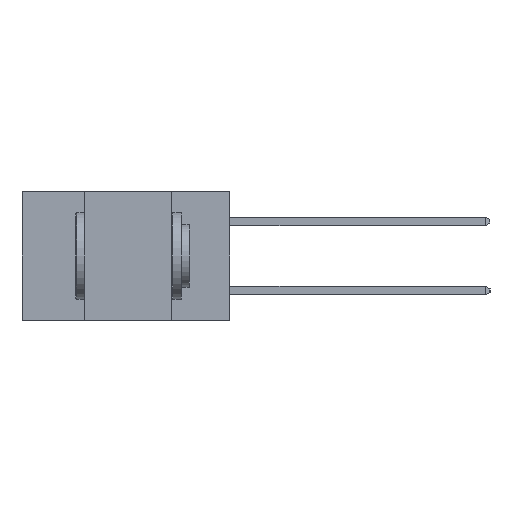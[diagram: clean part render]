
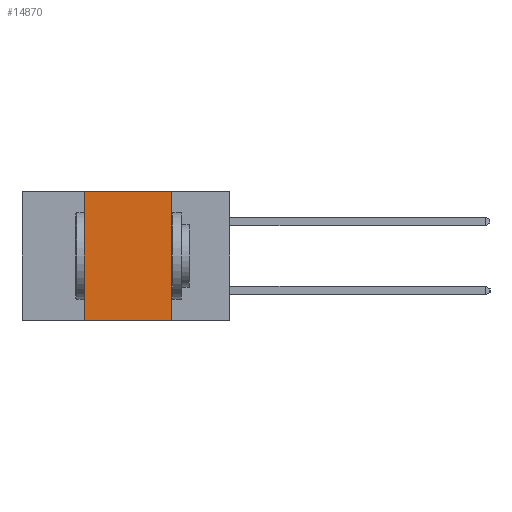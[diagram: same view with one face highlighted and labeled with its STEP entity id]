
A CAD part, left-side view. The second image highlights one B-rep face of the part: STEP entity #14870.
In plain terms, the highlighted planar face has unit normal (-1, 0, 0).
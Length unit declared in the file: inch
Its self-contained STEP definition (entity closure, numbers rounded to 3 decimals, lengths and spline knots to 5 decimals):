
#136 = CARTESIAN_POINT ( 'NONE',  ( 0., 0.6, 0. ) ) ;
#199 = LINE ( 'NONE', #8863, #11167 ) ;
#1555 = DIRECTION ( 'NONE',  ( 0., -1., 0. ) ) ;
#1939 = DIRECTION ( 'NONE',  ( 0., -1., 0. ) ) ;
#2019 = DIRECTION ( 'NONE',  ( 1., 0., 0. ) ) ;
#3711 = CARTESIAN_POINT ( 'NONE',  ( 0., 0.17, -0.37 ) ) ;
#3744 = ORIENTED_EDGE ( 'NONE', *, *, #12879, .F. ) ;
#4178 = FACE_OUTER_BOUND ( 'NONE', #18629, .T. ) ;
#4414 = LINE ( 'NONE', #15248, #24496 ) ;
#4954 = EDGE_CURVE ( 'NONE', #12142, #15135, #199, .T. ) ;
#5707 = CARTESIAN_POINT ( 'NONE',  ( 0., 0.17, 0. ) ) ;
#8863 = CARTESIAN_POINT ( 'NONE',  ( 0., 0.42, -0.37 ) ) ;
#8982 = LINE ( 'NONE', #3711, #13628 ) ;
#10090 = CARTESIAN_POINT ( 'NONE',  ( 0., 0.17, -0.37 ) ) ;
#10210 = EDGE_CURVE ( 'NONE', #12142, #16918, #4414, .T. ) ;
#10242 = AXIS2_PLACEMENT_3D ( 'NONE', #136, #2019, #15720 ) ;
#11167 = VECTOR ( 'NONE', #25030, 39.37008 ) ;
#11787 = PLANE ( 'NONE',  #10242 ) ;
#12142 = VERTEX_POINT ( 'NONE', #20817 ) ;
#12879 = EDGE_CURVE ( 'NONE', #15135, #16781, #23466, .T. ) ;
#13587 = ORIENTED_EDGE ( 'NONE', *, *, #18088, .F. ) ;
#13628 = VECTOR ( 'NONE', #15483, 39.37008 ) ;
#14186 = ORIENTED_EDGE ( 'NONE', *, *, #4954, .F. ) ;
#14870 = ADVANCED_FACE ( 'NONE', ( #4178 ), #11787, .F. ) ;
#15135 = VERTEX_POINT ( 'NONE', #24052 ) ;
#15248 = CARTESIAN_POINT ( 'NONE',  ( 0., 0.6, -0.37 ) ) ;
#15483 = DIRECTION ( 'NONE',  ( 0., 0., -1. ) ) ;
#15720 = DIRECTION ( 'NONE',  ( 0., 0., -1. ) ) ;
#16781 = VERTEX_POINT ( 'NONE', #5707 ) ;
#16918 = VERTEX_POINT ( 'NONE', #10090 ) ;
#17583 = CARTESIAN_POINT ( 'NONE',  ( 0., 0.6, 0. ) ) ;
#18088 = EDGE_CURVE ( 'NONE', #16781, #16918, #8982, .T. ) ;
#18629 = EDGE_LOOP ( 'NONE', ( #13587, #3744, #14186, #25023 ) ) ;
#20817 = CARTESIAN_POINT ( 'NONE',  ( 0., 0.42, -0.37 ) ) ;
#22877 = VECTOR ( 'NONE', #1939, 39.37008 ) ;
#23466 = LINE ( 'NONE', #17583, #22877 ) ;
#24052 = CARTESIAN_POINT ( 'NONE',  ( 0., 0.42, 0. ) ) ;
#24496 = VECTOR ( 'NONE', #1555, 39.37008 ) ;
#25023 = ORIENTED_EDGE ( 'NONE', *, *, #10210, .T. ) ;
#25030 = DIRECTION ( 'NONE',  ( 0., 0., 1. ) ) ;
